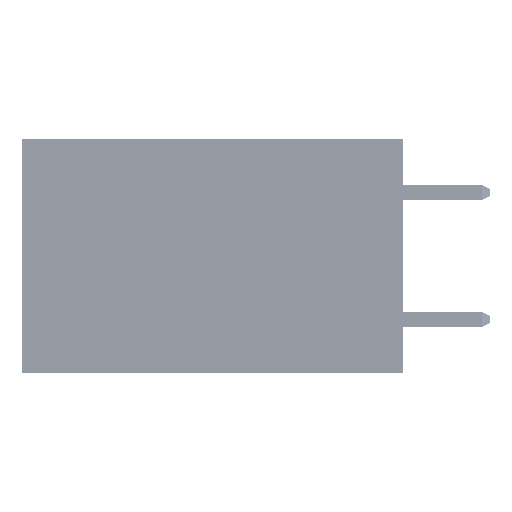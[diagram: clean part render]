
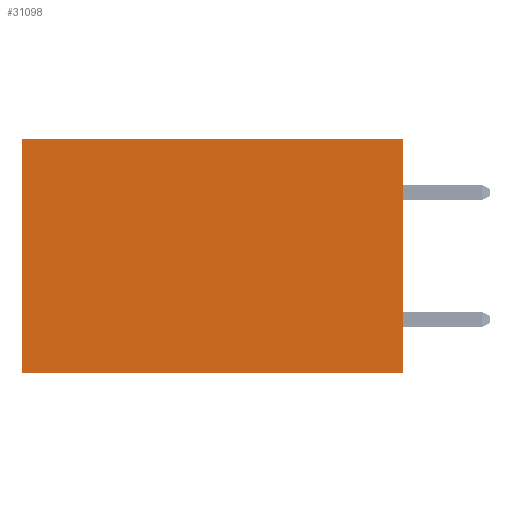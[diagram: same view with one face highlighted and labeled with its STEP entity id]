
A CAD part, left-side view. The second image highlights one B-rep face of the part: STEP entity #31098.
In plain terms, the highlighted planar face has unit normal (-1, 0, 0).
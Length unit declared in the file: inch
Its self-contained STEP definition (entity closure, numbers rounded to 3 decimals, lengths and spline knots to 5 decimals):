
#1528 = DIRECTION ( 'NONE',  ( 0., 1., 0. ) ) ;
#2778 = VECTOR ( 'NONE', #46811, 39.37008 ) ;
#5925 = DIRECTION ( 'NONE',  ( 0., 0., -1. ) ) ;
#6758 = EDGE_CURVE ( 'NONE', #28284, #51349, #45698, .T. ) ;
#7067 = CARTESIAN_POINT ( 'NONE',  ( 0.2875, 0.6, 0. ) ) ;
#8898 = CARTESIAN_POINT ( 'NONE',  ( 0.2875, 0., 0. ) ) ;
#11965 = ORIENTED_EDGE ( 'NONE', *, *, #45603, .T. ) ;
#13397 = VECTOR ( 'NONE', #47124, 39.37008 ) ;
#16303 = VERTEX_POINT ( 'NONE', #7067 ) ;
#17403 = DIRECTION ( 'NONE',  ( 0., 0., -1. ) ) ;
#17567 = VECTOR ( 'NONE', #5925, 39.37008 ) ;
#17570 = AXIS2_PLACEMENT_3D ( 'NONE', #41436, #17913, #17403 ) ;
#17913 = DIRECTION ( 'NONE',  ( 1., 0., 0. ) ) ;
#18839 = EDGE_LOOP ( 'NONE', ( #36802, #24436, #25119, #11965 ) ) ;
#22789 = CARTESIAN_POINT ( 'NONE',  ( 0.2875, 0., -0.37 ) ) ;
#24436 = ORIENTED_EDGE ( 'NONE', *, *, #6758, .F. ) ;
#25119 = ORIENTED_EDGE ( 'NONE', *, *, #35882, .F. ) ;
#25765 = LINE ( 'NONE', #8898, #17567 ) ;
#28284 = VERTEX_POINT ( 'NONE', #46401 ) ;
#29595 = PLANE ( 'NONE',  #17570 ) ;
#30012 = FACE_OUTER_BOUND ( 'NONE', #18839, .T. ) ;
#30787 = VERTEX_POINT ( 'NONE', #43572 ) ;
#31098 = ADVANCED_FACE ( 'NONE', ( #30012 ), #29595, .F. ) ;
#33622 = LINE ( 'NONE', #42532, #13397 ) ;
#35882 = EDGE_CURVE ( 'NONE', #30787, #28284, #25765, .T. ) ;
#36802 = ORIENTED_EDGE ( 'NONE', *, *, #38791, .T. ) ;
#38791 = EDGE_CURVE ( 'NONE', #16303, #51349, #33622, .T. ) ;
#40298 = VECTOR ( 'NONE', #1528, 39.37008 ) ;
#41436 = CARTESIAN_POINT ( 'NONE',  ( 0.2875, 0., 0. ) ) ;
#42532 = CARTESIAN_POINT ( 'NONE',  ( 0.2875, 0.6, 0. ) ) ;
#43572 = CARTESIAN_POINT ( 'NONE',  ( 0.2875, 0., 0. ) ) ;
#45603 = EDGE_CURVE ( 'NONE', #30787, #16303, #49860, .T. ) ;
#45698 = LINE ( 'NONE', #22789, #2778 ) ;
#46401 = CARTESIAN_POINT ( 'NONE',  ( 0.2875, 0., -0.37 ) ) ;
#46811 = DIRECTION ( 'NONE',  ( 0., 1., 0. ) ) ;
#47124 = DIRECTION ( 'NONE',  ( 0., 0., -1. ) ) ;
#49860 = LINE ( 'NONE', #50389, #40298 ) ;
#50389 = CARTESIAN_POINT ( 'NONE',  ( 0.2875, 0., 0. ) ) ;
#51349 = VERTEX_POINT ( 'NONE', #51582 ) ;
#51582 = CARTESIAN_POINT ( 'NONE',  ( 0.2875, 0.6, -0.37 ) ) ;
